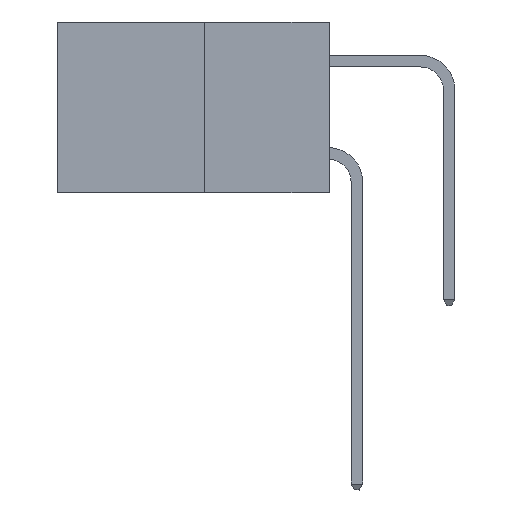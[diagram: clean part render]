
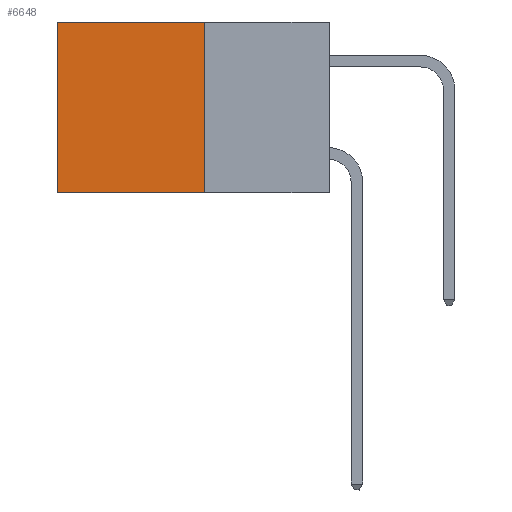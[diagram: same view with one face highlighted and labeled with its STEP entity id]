
A CAD part, left-side view. The second image highlights one B-rep face of the part: STEP entity #6648.
In plain terms, the highlighted planar face has unit normal (-1, 0, 0).
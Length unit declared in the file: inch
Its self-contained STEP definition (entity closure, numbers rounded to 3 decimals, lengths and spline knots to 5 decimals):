
#585 = CARTESIAN_POINT ( 'NONE',  ( 0.277, 0.27, -0.37 ) ) ;
#1477 = EDGE_CURVE ( 'NONE', #9163, #10632, #7965, .T. ) ;
#1671 = ORIENTED_EDGE ( 'NONE', *, *, #6769, .F. ) ;
#1754 = CARTESIAN_POINT ( 'NONE',  ( 0.277, 0.27, 0. ) ) ;
#1756 = DIRECTION ( 'NONE',  ( 0., 0., -1. ) ) ;
#2649 = DIRECTION ( 'NONE',  ( 0., 0., -1. ) ) ;
#3086 = VECTOR ( 'NONE', #4286, 39.37008 ) ;
#3452 = CARTESIAN_POINT ( 'NONE',  ( 0.277, 0.59, 0. ) ) ;
#3721 = CARTESIAN_POINT ( 'NONE',  ( 0.277, 0.27, -0.37 ) ) ;
#4286 = DIRECTION ( 'NONE',  ( 0., 0., -1. ) ) ;
#5101 = VERTEX_POINT ( 'NONE', #8602 ) ;
#5493 = LINE ( 'NONE', #11954, #11372 ) ;
#5961 = LINE ( 'NONE', #12424, #11848 ) ;
#6323 = PLANE ( 'NONE',  #13874 ) ;
#6534 = ORIENTED_EDGE ( 'NONE', *, *, #13802, .F. ) ;
#6648 = ADVANCED_FACE ( 'NONE', ( #10572 ), #6323, .F. ) ;
#6769 = EDGE_CURVE ( 'NONE', #7067, #5101, #5961, .T. ) ;
#7067 = VERTEX_POINT ( 'NONE', #3721 ) ;
#7075 = ORIENTED_EDGE ( 'NONE', *, *, #1477, .T. ) ;
#7453 = EDGE_CURVE ( 'NONE', #10632, #5101, #12351, .T. ) ;
#7600 = DIRECTION ( 'NONE',  ( 0., 1., 0. ) ) ;
#7965 = LINE ( 'NONE', #10481, #13790 ) ;
#8602 = CARTESIAN_POINT ( 'NONE',  ( 0.277, 0.59, -0.37 ) ) ;
#8680 = DIRECTION ( 'NONE',  ( 1., 0., 0. ) ) ;
#9143 = EDGE_LOOP ( 'NONE', ( #10555, #1671, #6534, #7075 ) ) ;
#9163 = VERTEX_POINT ( 'NONE', #1754 ) ;
#10481 = CARTESIAN_POINT ( 'NONE',  ( 0.277, 0.27, 0. ) ) ;
#10555 = ORIENTED_EDGE ( 'NONE', *, *, #7453, .T. ) ;
#10572 = FACE_OUTER_BOUND ( 'NONE', #9143, .T. ) ;
#10632 = VERTEX_POINT ( 'NONE', #3452 ) ;
#11372 = VECTOR ( 'NONE', #2649, 39.37008 ) ;
#11848 = VECTOR ( 'NONE', #13579, 39.37008 ) ;
#11954 = CARTESIAN_POINT ( 'NONE',  ( 0.277, 0.27, -0.37 ) ) ;
#12351 = LINE ( 'NONE', #14695, #3086 ) ;
#12424 = CARTESIAN_POINT ( 'NONE',  ( 0.277, 0.27, -0.37 ) ) ;
#13579 = DIRECTION ( 'NONE',  ( 0., 1., 0. ) ) ;
#13790 = VECTOR ( 'NONE', #7600, 39.37008 ) ;
#13802 = EDGE_CURVE ( 'NONE', #9163, #7067, #5493, .T. ) ;
#13874 = AXIS2_PLACEMENT_3D ( 'NONE', #585, #8680, #1756 ) ;
#14695 = CARTESIAN_POINT ( 'NONE',  ( 0.277, 0.59, -0.37 ) ) ;
